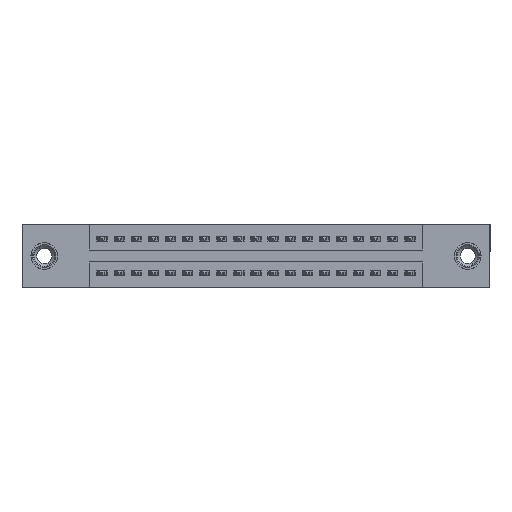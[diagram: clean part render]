
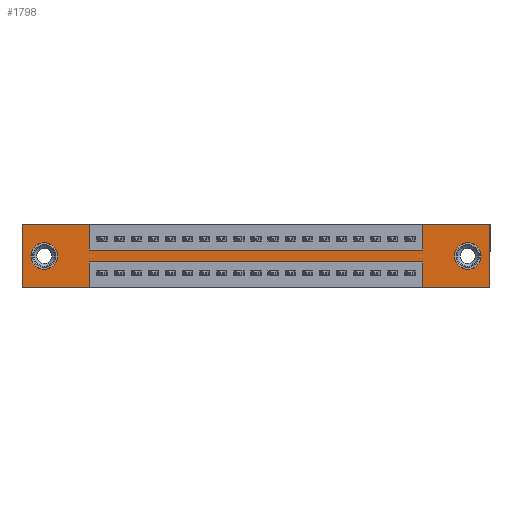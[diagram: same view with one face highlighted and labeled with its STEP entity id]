
A CAD part, front view. The second image highlights one B-rep face of the part: STEP entity #1798.
In plain terms, the highlighted planar face has unit normal (0, -1, 0).
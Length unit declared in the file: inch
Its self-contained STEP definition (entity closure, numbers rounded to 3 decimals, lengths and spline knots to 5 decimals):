
#77 = DIRECTION ( 'NONE',  ( 0., 0., -1. ) ) ;
#243 = VECTOR ( 'NONE', #7084, 39.37008 ) ;
#456 = CARTESIAN_POINT ( 'NONE',  ( 0.13, 0., -0.185 ) ) ;
#461 = CARTESIAN_POINT ( 'NONE',  ( 2.3425, 0., -0.37 ) ) ;
#565 = VECTOR ( 'NONE', #8843, 39.37008 ) ;
#930 = VERTEX_POINT ( 'NONE', #14391 ) ;
#1164 = CARTESIAN_POINT ( 'NONE',  ( 0.3925, 0., -0.15 ) ) ;
#1477 = VERTEX_POINT ( 'NONE', #1933 ) ;
#1723 = ORIENTED_EDGE ( 'NONE', *, *, #6662, .T. ) ;
#1798 = ADVANCED_FACE ( 'NONE', ( #11836, #3980, #20051 ), #17460, .T. ) ;
#1838 = VERTEX_POINT ( 'NONE', #13746 ) ;
#1933 = CARTESIAN_POINT ( 'NONE',  ( 0.3925, 0., -0.37 ) ) ;
#2006 = DIRECTION ( 'NONE',  ( 0., 0., 1. ) ) ;
#2009 = EDGE_CURVE ( 'NONE', #1477, #6604, #4205, .T. ) ;
#2223 = CARTESIAN_POINT ( 'NONE',  ( 2.605, 0., -0.185 ) ) ;
#2428 = VECTOR ( 'NONE', #19640, 39.37008 ) ;
#2583 = CARTESIAN_POINT ( 'NONE',  ( 2.735, 0., 0. ) ) ;
#2587 = VERTEX_POINT ( 'NONE', #13864 ) ;
#2646 = AXIS2_PLACEMENT_3D ( 'NONE', #2223, #13198, #3798 ) ;
#2677 = EDGE_LOOP ( 'NONE', ( #5010, #16934, #17935, #16070, #9470, #5698, #14938, #18077, #14530, #10218, #13747, #11696 ) ) ;
#2745 = DIRECTION ( 'NONE',  ( 1., 0., 0. ) ) ;
#2883 = CARTESIAN_POINT ( 'NONE',  ( 2.735, 0., -0.37 ) ) ;
#2892 = CARTESIAN_POINT ( 'NONE',  ( 0.13, 0., -0.263 ) ) ;
#2986 = CIRCLE ( 'NONE', #13990, 0.078 ) ;
#3173 = EDGE_CURVE ( 'NONE', #14111, #14063, #3923, .T. ) ;
#3440 = CARTESIAN_POINT ( 'NONE',  ( 2.605, 0., -0.185 ) ) ;
#3677 = CARTESIAN_POINT ( 'NONE',  ( 0.3925, 0., 0. ) ) ;
#3798 = DIRECTION ( 'NONE',  ( 0., 0., -1. ) ) ;
#3907 = DIRECTION ( 'NONE',  ( 0., 0., 1. ) ) ;
#3923 = LINE ( 'NONE', #4977, #243 ) ;
#3980 = FACE_BOUND ( 'NONE', #14739, .T. ) ;
#4056 = EDGE_CURVE ( 'NONE', #2587, #4429, #19959, .T. ) ;
#4151 = EDGE_CURVE ( 'NONE', #1838, #4240, #10729, .T. ) ;
#4205 = LINE ( 'NONE', #5308, #8893 ) ;
#4240 = VERTEX_POINT ( 'NONE', #10224 ) ;
#4289 = CIRCLE ( 'NONE', #14904, 0.078 ) ;
#4429 = VERTEX_POINT ( 'NONE', #2892 ) ;
#4496 = DIRECTION ( 'NONE',  ( 0., 1., 0. ) ) ;
#4638 = DIRECTION ( 'NONE',  ( 0., 0., -1. ) ) ;
#4844 = DIRECTION ( 'NONE',  ( 0., 0., -1. ) ) ;
#4912 = EDGE_CURVE ( 'NONE', #10373, #5929, #18512, .T. ) ;
#4977 = CARTESIAN_POINT ( 'NONE',  ( 0., 0., 0. ) ) ;
#5010 = ORIENTED_EDGE ( 'NONE', *, *, #19218, .F. ) ;
#5027 = CARTESIAN_POINT ( 'NONE',  ( 2.3425, 0., -0.15 ) ) ;
#5069 = DIRECTION ( 'NONE',  ( 0., 0., -1. ) ) ;
#5166 = CARTESIAN_POINT ( 'NONE',  ( 0., 0., -0.37 ) ) ;
#5308 = CARTESIAN_POINT ( 'NONE',  ( 0., 0., -0.37 ) ) ;
#5378 = ORIENTED_EDGE ( 'NONE', *, *, #14421, .T. ) ;
#5698 = ORIENTED_EDGE ( 'NONE', *, *, #3173, .F. ) ;
#5714 = CARTESIAN_POINT ( 'NONE',  ( 2.3425, 0., 0. ) ) ;
#5929 = VERTEX_POINT ( 'NONE', #12637 ) ;
#6040 = EDGE_CURVE ( 'NONE', #6604, #930, #14131, .T. ) ;
#6322 = LINE ( 'NONE', #17346, #14154 ) ;
#6604 = VERTEX_POINT ( 'NONE', #13737 ) ;
#6611 = LINE ( 'NONE', #15062, #2428 ) ;
#6662 = EDGE_CURVE ( 'NONE', #4429, #2587, #4289, .T. ) ;
#7042 = EDGE_LOOP ( 'NONE', ( #5378, #7612 ) ) ;
#7053 = DIRECTION ( 'NONE',  ( -1., 0., 0. ) ) ;
#7084 = DIRECTION ( 'NONE',  ( 1., 0., 0. ) ) ;
#7612 = ORIENTED_EDGE ( 'NONE', *, *, #4151, .T. ) ;
#8085 = VERTEX_POINT ( 'NONE', #13970 ) ;
#8335 = VERTEX_POINT ( 'NONE', #3677 ) ;
#8595 = LINE ( 'NONE', #1164, #16389 ) ;
#8675 = VECTOR ( 'NONE', #7053, 39.37008 ) ;
#8818 = VECTOR ( 'NONE', #4638, 39.37008 ) ;
#8843 = DIRECTION ( 'NONE',  ( 0., 0., 1. ) ) ;
#8871 = VECTOR ( 'NONE', #12628, 39.37008 ) ;
#8893 = VECTOR ( 'NONE', #9896, 39.37008 ) ;
#8969 = EDGE_CURVE ( 'NONE', #5929, #15971, #9160, .T. ) ;
#9160 = LINE ( 'NONE', #10165, #8675 ) ;
#9295 = LINE ( 'NONE', #18667, #8818 ) ;
#9470 = ORIENTED_EDGE ( 'NONE', *, *, #12117, .F. ) ;
#9656 = VERTEX_POINT ( 'NONE', #5027 ) ;
#9744 = DIRECTION ( 'NONE',  ( 0., 0., 1. ) ) ;
#9896 = DIRECTION ( 'NONE',  ( -1., 0., 0. ) ) ;
#9911 = EDGE_CURVE ( 'NONE', #9656, #14111, #13072, .T. ) ;
#9954 = VECTOR ( 'NONE', #9744, 39.37008 ) ;
#9965 = ORIENTED_EDGE ( 'NONE', *, *, #4056, .T. ) ;
#10165 = CARTESIAN_POINT ( 'NONE',  ( 0.3925, 0., -0.22 ) ) ;
#10169 = LINE ( 'NONE', #18774, #18433 ) ;
#10218 = ORIENTED_EDGE ( 'NONE', *, *, #10811, .F. ) ;
#10224 = CARTESIAN_POINT ( 'NONE',  ( 2.605, 0., -0.107 ) ) ;
#10373 = VERTEX_POINT ( 'NONE', #461 ) ;
#10729 = CIRCLE ( 'NONE', #2646, 0.078 ) ;
#10811 = EDGE_CURVE ( 'NONE', #930, #8335, #13026, .T. ) ;
#11421 = DIRECTION ( 'NONE',  ( 0., 1., 0. ) ) ;
#11696 = ORIENTED_EDGE ( 'NONE', *, *, #2009, .F. ) ;
#11836 = FACE_BOUND ( 'NONE', #7042, .T. ) ;
#12117 = EDGE_CURVE ( 'NONE', #14063, #15760, #9295, .T. ) ;
#12628 = DIRECTION ( 'NONE',  ( 1., 0., 0. ) ) ;
#12637 = CARTESIAN_POINT ( 'NONE',  ( 2.3425, 0., -0.22 ) ) ;
#13026 = LINE ( 'NONE', #17244, #8871 ) ;
#13072 = LINE ( 'NONE', #5714, #565 ) ;
#13198 = DIRECTION ( 'NONE',  ( 0., 1., 0. ) ) ;
#13737 = CARTESIAN_POINT ( 'NONE',  ( 0., 0., -0.37 ) ) ;
#13746 = CARTESIAN_POINT ( 'NONE',  ( 2.605, 0., -0.263 ) ) ;
#13747 = ORIENTED_EDGE ( 'NONE', *, *, #6040, .F. ) ;
#13864 = CARTESIAN_POINT ( 'NONE',  ( 0.13, 0., -0.107 ) ) ;
#13884 = CARTESIAN_POINT ( 'NONE',  ( 0.13, 0., -0.185 ) ) ;
#13970 = CARTESIAN_POINT ( 'NONE',  ( 0.3925, 0., -0.15 ) ) ;
#13990 = AXIS2_PLACEMENT_3D ( 'NONE', #3440, #14431, #5069 ) ;
#14063 = VERTEX_POINT ( 'NONE', #2583 ) ;
#14111 = VERTEX_POINT ( 'NONE', #19815 ) ;
#14131 = LINE ( 'NONE', #15974, #9954 ) ;
#14154 = VECTOR ( 'NONE', #18887, 39.37008 ) ;
#14391 = CARTESIAN_POINT ( 'NONE',  ( 0., 0., 0. ) ) ;
#14421 = EDGE_CURVE ( 'NONE', #4240, #1838, #2986, .T. ) ;
#14431 = DIRECTION ( 'NONE',  ( 0., 1., 0. ) ) ;
#14436 = VECTOR ( 'NONE', #3907, 39.37008 ) ;
#14530 = ORIENTED_EDGE ( 'NONE', *, *, #16225, .F. ) ;
#14739 = EDGE_LOOP ( 'NONE', ( #9965, #1723 ) ) ;
#14904 = AXIS2_PLACEMENT_3D ( 'NONE', #13884, #4496, #15440 ) ;
#14938 = ORIENTED_EDGE ( 'NONE', *, *, #9911, .F. ) ;
#15062 = CARTESIAN_POINT ( 'NONE',  ( 0.3925, 0., 0. ) ) ;
#15440 = DIRECTION ( 'NONE',  ( 0., 0., 1. ) ) ;
#15681 = EDGE_CURVE ( 'NONE', #8085, #9656, #8595, .T. ) ;
#15760 = VERTEX_POINT ( 'NONE', #2883 ) ;
#15875 = CARTESIAN_POINT ( 'NONE',  ( 0.3925, 0., -0.22 ) ) ;
#15971 = VERTEX_POINT ( 'NONE', #15875 ) ;
#15974 = CARTESIAN_POINT ( 'NONE',  ( 0., 0., 0. ) ) ;
#16070 = ORIENTED_EDGE ( 'NONE', *, *, #19927, .F. ) ;
#16225 = EDGE_CURVE ( 'NONE', #8335, #8085, #6611, .T. ) ;
#16389 = VECTOR ( 'NONE', #2745, 39.37008 ) ;
#16923 = DIRECTION ( 'NONE',  ( 0., -1., 0. ) ) ;
#16934 = ORIENTED_EDGE ( 'NONE', *, *, #8969, .F. ) ;
#17244 = CARTESIAN_POINT ( 'NONE',  ( 0., 0., 0. ) ) ;
#17346 = CARTESIAN_POINT ( 'NONE',  ( 0., 0., -0.37 ) ) ;
#17460 = PLANE ( 'NONE',  #18294 ) ;
#17702 = AXIS2_PLACEMENT_3D ( 'NONE', #456, #11421, #2006 ) ;
#17935 = ORIENTED_EDGE ( 'NONE', *, *, #4912, .F. ) ;
#18077 = ORIENTED_EDGE ( 'NONE', *, *, #15681, .F. ) ;
#18294 = AXIS2_PLACEMENT_3D ( 'NONE', #5166, #16923, #4844 ) ;
#18433 = VECTOR ( 'NONE', #77, 39.37008 ) ;
#18512 = LINE ( 'NONE', #19440, #14436 ) ;
#18667 = CARTESIAN_POINT ( 'NONE',  ( 2.735, 0., 0. ) ) ;
#18774 = CARTESIAN_POINT ( 'NONE',  ( 0.3925, 0., -0.37 ) ) ;
#18887 = DIRECTION ( 'NONE',  ( -1., 0., 0. ) ) ;
#19218 = EDGE_CURVE ( 'NONE', #15971, #1477, #10169, .T. ) ;
#19440 = CARTESIAN_POINT ( 'NONE',  ( 2.3425, 0., -0.37 ) ) ;
#19640 = DIRECTION ( 'NONE',  ( 0., 0., -1. ) ) ;
#19815 = CARTESIAN_POINT ( 'NONE',  ( 2.3425, 0., 0. ) ) ;
#19927 = EDGE_CURVE ( 'NONE', #15760, #10373, #6322, .T. ) ;
#19959 = CIRCLE ( 'NONE', #17702, 0.078 ) ;
#20051 = FACE_OUTER_BOUND ( 'NONE', #2677, .T. ) ;
